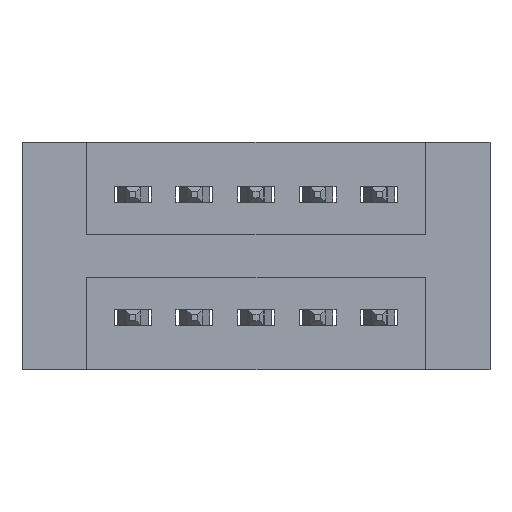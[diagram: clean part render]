
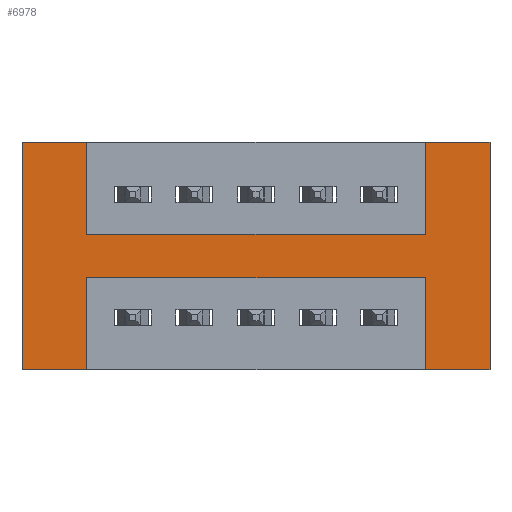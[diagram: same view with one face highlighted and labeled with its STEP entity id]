
A CAD part, front view. The second image highlights one B-rep face of the part: STEP entity #6978.
In plain terms, the highlighted planar face has unit normal (0, -1, 0).
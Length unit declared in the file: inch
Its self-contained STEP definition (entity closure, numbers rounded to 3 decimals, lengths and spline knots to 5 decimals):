
#214 = PLANE ( 'NONE',  #6962 ) ;
#308 = EDGE_CURVE ( 'NONE', #2289, #7652, #4814, .T. ) ;
#315 = VECTOR ( 'NONE', #8310, 39.37008 ) ;
#326 = VERTEX_POINT ( 'NONE', #4064 ) ;
#590 = CARTESIAN_POINT ( 'NONE',  ( 0.3925, 0., -0.15 ) ) ;
#606 = ORIENTED_EDGE ( 'NONE', *, *, #4850, .F. ) ;
#632 = CARTESIAN_POINT ( 'NONE',  ( 0.9425, 0., -0.37 ) ) ;
#780 = VERTEX_POINT ( 'NONE', #7465 ) ;
#803 = EDGE_CURVE ( 'NONE', #7428, #2289, #3405, .T. ) ;
#927 = VERTEX_POINT ( 'NONE', #2603 ) ;
#997 = VECTOR ( 'NONE', #1805, 39.37008 ) ;
#1014 = CARTESIAN_POINT ( 'NONE',  ( 0.3925, 0., -0.37 ) ) ;
#1080 = ORIENTED_EDGE ( 'NONE', *, *, #803, .F. ) ;
#1141 = CARTESIAN_POINT ( 'NONE',  ( 0.9425, 0., -0.37 ) ) ;
#1168 = DIRECTION ( 'NONE',  ( 1., 0., 0. ) ) ;
#1173 = LINE ( 'NONE', #3341, #315 ) ;
#1273 = VECTOR ( 'NONE', #7635, 39.37008 ) ;
#1295 = DIRECTION ( 'NONE',  ( -1., 0., 0. ) ) ;
#1355 = CARTESIAN_POINT ( 'NONE',  ( 1.0475, 0., 0. ) ) ;
#1377 = EDGE_CURVE ( 'NONE', #2080, #780, #7036, .T. ) ;
#1383 = ORIENTED_EDGE ( 'NONE', *, *, #6937, .T. ) ;
#1412 = CARTESIAN_POINT ( 'NONE',  ( 0., 0., -0.37 ) ) ;
#1549 = EDGE_CURVE ( 'NONE', #7652, #326, #1720, .T. ) ;
#1655 = CARTESIAN_POINT ( 'NONE',  ( 0.2875, 0., 0. ) ) ;
#1720 = LINE ( 'NONE', #6221, #8287 ) ;
#1748 = LINE ( 'NONE', #3252, #8608 ) ;
#1805 = DIRECTION ( 'NONE',  ( -1., 0., 0. ) ) ;
#2080 = VERTEX_POINT ( 'NONE', #3907 ) ;
#2121 = LINE ( 'NONE', #3382, #2646 ) ;
#2258 = CARTESIAN_POINT ( 'NONE',  ( 0., 0., -0.37 ) ) ;
#2289 = VERTEX_POINT ( 'NONE', #632 ) ;
#2382 = EDGE_CURVE ( 'NONE', #780, #6845, #1173, .T. ) ;
#2401 = VECTOR ( 'NONE', #6921, 39.37008 ) ;
#2518 = ORIENTED_EDGE ( 'NONE', *, *, #1377, .F. ) ;
#2603 = CARTESIAN_POINT ( 'NONE',  ( 0.3925, 0., -0.37 ) ) ;
#2613 = LINE ( 'NONE', #7172, #8154 ) ;
#2646 = VECTOR ( 'NONE', #8607, 39.37008 ) ;
#2689 = EDGE_CURVE ( 'NONE', #3004, #2816, #2613, .T. ) ;
#2816 = VERTEX_POINT ( 'NONE', #3522 ) ;
#2830 = CARTESIAN_POINT ( 'NONE',  ( 0.9425, 0., -0.15 ) ) ;
#3004 = VERTEX_POINT ( 'NONE', #6610 ) ;
#3252 = CARTESIAN_POINT ( 'NONE',  ( 0.9425, 0., 0. ) ) ;
#3341 = CARTESIAN_POINT ( 'NONE',  ( 0.3925, 0., 0. ) ) ;
#3347 = DIRECTION ( 'NONE',  ( 0., 0., 1. ) ) ;
#3350 = ORIENTED_EDGE ( 'NONE', *, *, #8656, .F. ) ;
#3382 = CARTESIAN_POINT ( 'NONE',  ( 0.3925, 0., -0.15 ) ) ;
#3405 = LINE ( 'NONE', #1412, #997 ) ;
#3434 = EDGE_CURVE ( 'NONE', #2080, #6997, #7748, .T. ) ;
#3522 = CARTESIAN_POINT ( 'NONE',  ( 1.0475, 0., 0. ) ) ;
#3595 = DIRECTION ( 'NONE',  ( 0., 0., -1. ) ) ;
#3907 = CARTESIAN_POINT ( 'NONE',  ( 0.2875, 0., 0. ) ) ;
#4064 = CARTESIAN_POINT ( 'NONE',  ( 0.3925, 0., -0.22 ) ) ;
#4282 = CARTESIAN_POINT ( 'NONE',  ( 0.2875, 0., -0.37 ) ) ;
#4313 = LINE ( 'NONE', #1014, #1273 ) ;
#4601 = CARTESIAN_POINT ( 'NONE',  ( 0.9425, 0., -0.22 ) ) ;
#4814 = LINE ( 'NONE', #1141, #8406 ) ;
#4834 = LINE ( 'NONE', #5964, #6658 ) ;
#4850 = EDGE_CURVE ( 'NONE', #326, #927, #4313, .T. ) ;
#4967 = CARTESIAN_POINT ( 'NONE',  ( 1.0475, 0., -0.37 ) ) ;
#5070 = DIRECTION ( 'NONE',  ( 0., -1., 0. ) ) ;
#5167 = EDGE_LOOP ( 'NONE', ( #1383, #7687, #5642, #3350, #6113, #2518, #6535, #8544, #606, #8392, #5860, #1080 ) ) ;
#5217 = DIRECTION ( 'NONE',  ( 1., 0., 0. ) ) ;
#5642 = ORIENTED_EDGE ( 'NONE', *, *, #7658, .F. ) ;
#5844 = DIRECTION ( 'NONE',  ( 0., 0., 1. ) ) ;
#5860 = ORIENTED_EDGE ( 'NONE', *, *, #308, .F. ) ;
#5943 = LINE ( 'NONE', #1355, #8115 ) ;
#5964 = CARTESIAN_POINT ( 'NONE',  ( 0., 0., -0.37 ) ) ;
#6113 = ORIENTED_EDGE ( 'NONE', *, *, #2382, .F. ) ;
#6221 = CARTESIAN_POINT ( 'NONE',  ( 0.3925, 0., -0.22 ) ) ;
#6535 = ORIENTED_EDGE ( 'NONE', *, *, #3434, .T. ) ;
#6610 = CARTESIAN_POINT ( 'NONE',  ( 0.9425, 0., 0. ) ) ;
#6658 = VECTOR ( 'NONE', #1295, 39.37008 ) ;
#6805 = EDGE_CURVE ( 'NONE', #927, #6997, #4834, .T. ) ;
#6845 = VERTEX_POINT ( 'NONE', #590 ) ;
#6921 = DIRECTION ( 'NONE',  ( 0., 0., -1. ) ) ;
#6937 = EDGE_CURVE ( 'NONE', #7428, #2816, #5943, .T. ) ;
#6962 = AXIS2_PLACEMENT_3D ( 'NONE', #2258, #5070, #3595 ) ;
#6978 = ADVANCED_FACE ( 'NONE', ( #8518 ), #214, .T. ) ;
#6997 = VERTEX_POINT ( 'NONE', #4282 ) ;
#7036 = LINE ( 'NONE', #7131, #7564 ) ;
#7131 = CARTESIAN_POINT ( 'NONE',  ( 0., 0., 0. ) ) ;
#7172 = CARTESIAN_POINT ( 'NONE',  ( 0., 0., 0. ) ) ;
#7385 = DIRECTION ( 'NONE',  ( 0., 0., 1. ) ) ;
#7428 = VERTEX_POINT ( 'NONE', #4967 ) ;
#7465 = CARTESIAN_POINT ( 'NONE',  ( 0.3925, 0., 0. ) ) ;
#7564 = VECTOR ( 'NONE', #5217, 39.37008 ) ;
#7635 = DIRECTION ( 'NONE',  ( 0., 0., -1. ) ) ;
#7652 = VERTEX_POINT ( 'NONE', #4601 ) ;
#7658 = EDGE_CURVE ( 'NONE', #8313, #3004, #1748, .T. ) ;
#7687 = ORIENTED_EDGE ( 'NONE', *, *, #2689, .F. ) ;
#7748 = LINE ( 'NONE', #1655, #2401 ) ;
#8115 = VECTOR ( 'NONE', #7385, 39.37008 ) ;
#8154 = VECTOR ( 'NONE', #1168, 39.37008 ) ;
#8244 = DIRECTION ( 'NONE',  ( -1., 0., 0. ) ) ;
#8287 = VECTOR ( 'NONE', #8244, 39.37008 ) ;
#8310 = DIRECTION ( 'NONE',  ( 0., 0., -1. ) ) ;
#8313 = VERTEX_POINT ( 'NONE', #2830 ) ;
#8392 = ORIENTED_EDGE ( 'NONE', *, *, #1549, .F. ) ;
#8406 = VECTOR ( 'NONE', #5844, 39.37008 ) ;
#8518 = FACE_OUTER_BOUND ( 'NONE', #5167, .T. ) ;
#8544 = ORIENTED_EDGE ( 'NONE', *, *, #6805, .F. ) ;
#8607 = DIRECTION ( 'NONE',  ( 1., 0., 0. ) ) ;
#8608 = VECTOR ( 'NONE', #3347, 39.37008 ) ;
#8656 = EDGE_CURVE ( 'NONE', #6845, #8313, #2121, .T. ) ;
